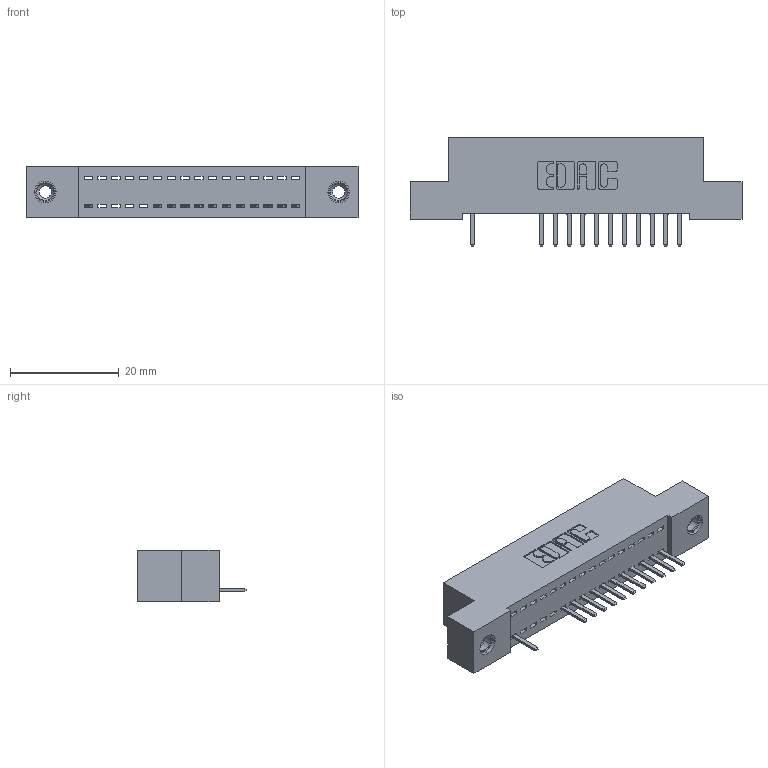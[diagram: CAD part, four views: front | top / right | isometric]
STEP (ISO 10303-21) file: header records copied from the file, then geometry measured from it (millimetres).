
FILE_DESCRIPTION (( 'STEP AP203' ), '1' );
FILE_NAME ('392-016-520-108.STEP', '2018-08-15T01:22:13', ( '' ), ( '' ), 'SwSTEP 2.0', 'SolidWorks 2016', '' );
FILE_SCHEMA (( 'CONFIG_CONTROL_DESIGN' ));
Length unit declared in the file: inch
Products named in the file (4): 345-292-001_345-293-120; 345-250-001_345-250-003-102; 392-016-520-108; 342 Part_TI
Assembly tree (15 placements, depth 2):
  392-016-520-108
    342 Part_TI
    345-292-001_345-293-120  x12
    345-250-001_345-250-003-102  x2
Bounding box: 60.96 x 20.02 x 9.4 mm (x, y, z)
Volume: 5163.3 mm3; surface area: 6766.9 mm2
Topology: 15 solids, 15 shells, 962 faces, 2811 edges, 1834 vertices
Faces by surface type: plane 674, cylinder 272, cone 12, torus 4
Entity records: 14184 total; most frequent: CARTESIAN_POINT 2461, ORIENTED_EDGE 2398, DIRECTION 2145, EDGE_CURVE 1199, LINE 1047, VECTOR 1047, VERTEX_POINT 792, AXIS2_PLACEMENT_3D 549
